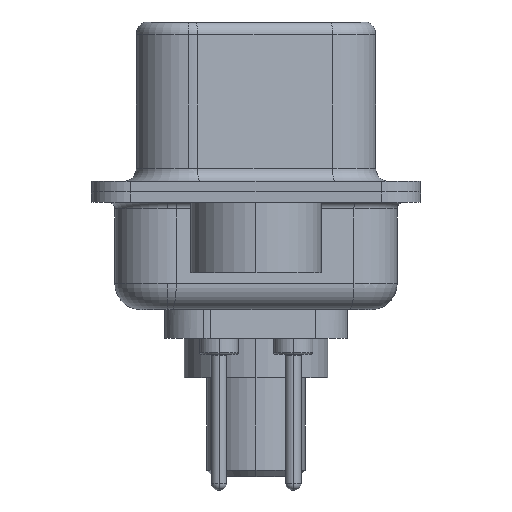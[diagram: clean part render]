
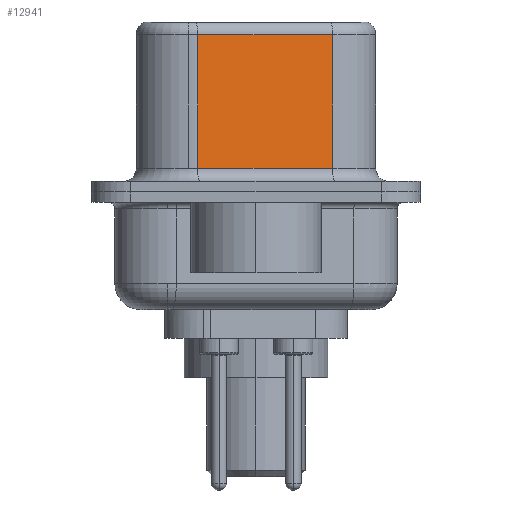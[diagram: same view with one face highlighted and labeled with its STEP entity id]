
A CAD part, left-side view. The second image highlights one B-rep face of the part: STEP entity #12941.
In plain terms, the highlighted planar face has unit normal (-0.985, -0.174, 0).
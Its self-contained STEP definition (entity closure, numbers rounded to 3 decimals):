
#997 = EDGE_CURVE ( 'NONE', #7416, #10780, #6137, .T. ) ;
#1315 = CARTESIAN_POINT ( 'NONE',  ( 4.58, -2.927, 6.02 ) ) ;
#1606 = CARTESIAN_POINT ( 'NONE',  ( 4.58, -2.927, 0.9 ) ) ;
#1764 = EDGE_LOOP ( 'NONE', ( #14024, #8252, #4017, #7159 ) ) ;
#1793 = LINE ( 'NONE', #1606, #10066 ) ;
#2340 = EDGE_CURVE ( 'NONE', #7416, #10921, #2456, .T. ) ;
#2456 = LINE ( 'NONE', #10349, #10698 ) ;
#2544 = CARTESIAN_POINT ( 'NONE',  ( 3.67, 2.233, 0.9 ) ) ;
#2697 = FACE_OUTER_BOUND ( 'NONE', #1764, .T. ) ;
#3262 = LINE ( 'NONE', #10197, #11438 ) ;
#3590 = DIRECTION ( 'NONE',  ( -0.174, 0.985, 0. ) ) ;
#3988 = VECTOR ( 'NONE', #10677, 1000. ) ;
#4017 = ORIENTED_EDGE ( 'NONE', *, *, #4831, .T. ) ;
#4831 = EDGE_CURVE ( 'NONE', #10780, #5469, #3262, .T. ) ;
#5469 = VERTEX_POINT ( 'NONE', #2544 ) ;
#6137 = LINE ( 'NONE', #1315, #3988 ) ;
#6713 = EDGE_CURVE ( 'NONE', #5469, #10921, #1793, .T. ) ;
#7159 = ORIENTED_EDGE ( 'NONE', *, *, #6713, .T. ) ;
#7416 = VERTEX_POINT ( 'NONE', #11153 ) ;
#7759 = DIRECTION ( 'NONE',  ( 0.174, -0.985, 0. ) ) ;
#7876 = PLANE ( 'NONE',  #13946 ) ;
#8252 = ORIENTED_EDGE ( 'NONE', *, *, #997, .T. ) ;
#8734 = DIRECTION ( 'NONE',  ( 0., 0., -1. ) ) ;
#8977 = CARTESIAN_POINT ( 'NONE',  ( 4.58, -2.927, 6.52 ) ) ;
#9770 = CARTESIAN_POINT ( 'NONE',  ( 4.58, -2.927, 0.9 ) ) ;
#10012 = DIRECTION ( 'NONE',  ( 0.985, 0.174, 0. ) ) ;
#10066 = VECTOR ( 'NONE', #7759, 1000. ) ;
#10197 = CARTESIAN_POINT ( 'NONE',  ( 3.67, 2.233, 6.52 ) ) ;
#10349 = CARTESIAN_POINT ( 'NONE',  ( 4.58, -2.927, 6.52 ) ) ;
#10627 = CARTESIAN_POINT ( 'NONE',  ( 3.67, 2.233, 6.02 ) ) ;
#10677 = DIRECTION ( 'NONE',  ( -0.174, 0.985, 0. ) ) ;
#10698 = VECTOR ( 'NONE', #8734, 1000. ) ;
#10780 = VERTEX_POINT ( 'NONE', #10627 ) ;
#10921 = VERTEX_POINT ( 'NONE', #9770 ) ;
#10998 = DIRECTION ( 'NONE',  ( 0., 0., -1. ) ) ;
#11153 = CARTESIAN_POINT ( 'NONE',  ( 4.58, -2.927, 6.02 ) ) ;
#11438 = VECTOR ( 'NONE', #10998, 1000. ) ;
#12941 = ADVANCED_FACE ( 'NONE', ( #2697 ), #7876, .F. ) ;
#13946 = AXIS2_PLACEMENT_3D ( 'NONE', #8977, #10012, #3590 ) ;
#14024 = ORIENTED_EDGE ( 'NONE', *, *, #2340, .F. ) ;
